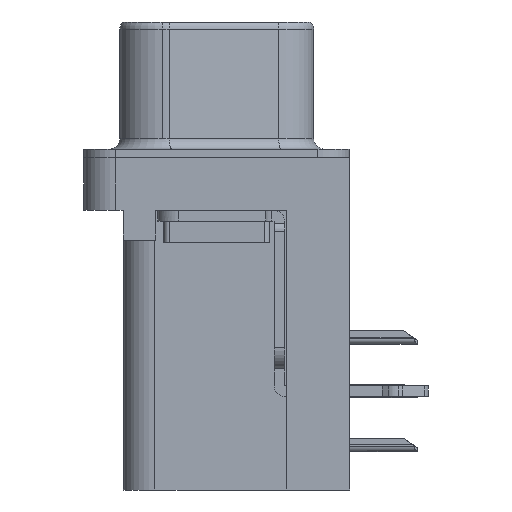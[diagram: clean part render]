
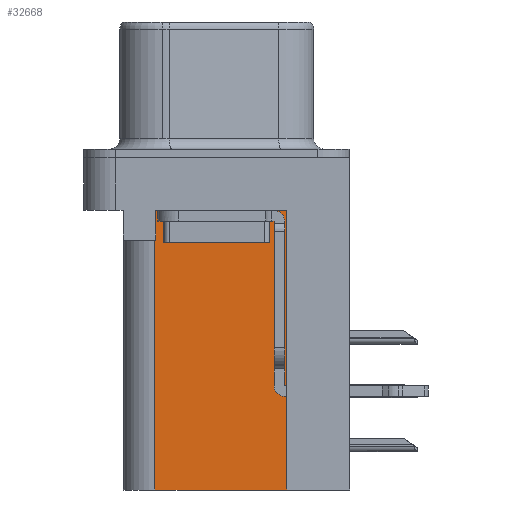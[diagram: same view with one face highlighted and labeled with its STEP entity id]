
A CAD part, left-side view. The second image highlights one B-rep face of the part: STEP entity #32668.
In plain terms, the highlighted planar face has unit normal (-1, 0, 0).
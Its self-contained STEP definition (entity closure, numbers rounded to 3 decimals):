
#428 = DIRECTION ( 'NONE',  ( 0., 1., 0. ) ) ;
#1428 = DIRECTION ( 'NONE',  ( 0., 1., 0. ) ) ;
#2313 = LINE ( 'NONE', #2747, #16010 ) ;
#2744 = CARTESIAN_POINT ( 'NONE',  ( 3.79, 2.895, -3.9 ) ) ;
#2747 = CARTESIAN_POINT ( 'NONE',  ( 3.79, 2.925, -15.7 ) ) ;
#3429 = DIRECTION ( 'NONE',  ( 0., 1., 0. ) ) ;
#3838 = VECTOR ( 'NONE', #3429, 1000. ) ;
#4020 = CARTESIAN_POINT ( 'NONE',  ( 3.79, -3.295, -15.7 ) ) ;
#4202 = EDGE_LOOP ( 'NONE', ( #34467, #12110, #12294, #6797, #34744, #28537 ) ) ;
#4486 = VERTEX_POINT ( 'NONE', #23961 ) ;
#4537 = AXIS2_PLACEMENT_3D ( 'NONE', #4020, #26140, #9547 ) ;
#5960 = VECTOR ( 'NONE', #428, 1000. ) ;
#6689 = CARTESIAN_POINT ( 'NONE',  ( 3.79, 2.895, -3.9 ) ) ;
#6797 = ORIENTED_EDGE ( 'NONE', *, *, #20792, .F. ) ;
#6993 = LINE ( 'NONE', #6689, #27405 ) ;
#8713 = VERTEX_POINT ( 'NONE', #30419 ) ;
#9253 = FACE_OUTER_BOUND ( 'NONE', #4202, .T. ) ;
#9378 = DIRECTION ( 'NONE',  ( 0., 0., -1. ) ) ;
#9547 = DIRECTION ( 'NONE',  ( 0., 0., -1. ) ) ;
#10497 = DIRECTION ( 'NONE',  ( 0., 0., 1. ) ) ;
#10613 = CARTESIAN_POINT ( 'NONE',  ( 3.79, -3.295, -15.7 ) ) ;
#11986 = LINE ( 'NONE', #17105, #3838 ) ;
#12110 = ORIENTED_EDGE ( 'NONE', *, *, #25932, .T. ) ;
#12294 = ORIENTED_EDGE ( 'NONE', *, *, #30593, .T. ) ;
#13879 = CARTESIAN_POINT ( 'NONE',  ( 3.79, 2.895, -2.5 ) ) ;
#14132 = VECTOR ( 'NONE', #1428, 1000. ) ;
#14515 = VERTEX_POINT ( 'NONE', #21530 ) ;
#15463 = LINE ( 'NONE', #10613, #22003 ) ;
#16010 = VECTOR ( 'NONE', #35980, 1000. ) ;
#16483 = CARTESIAN_POINT ( 'NONE',  ( 3.79, -3.295, -2.5 ) ) ;
#16858 = CARTESIAN_POINT ( 'NONE',  ( 3.79, -3.295, -15.7 ) ) ;
#17105 = CARTESIAN_POINT ( 'NONE',  ( 3.79, 0., -3.9 ) ) ;
#17711 = PLANE ( 'NONE',  #4537 ) ;
#17827 = CARTESIAN_POINT ( 'NONE',  ( 3.79, -3.295, -2.5 ) ) ;
#19565 = VERTEX_POINT ( 'NONE', #16483 ) ;
#20792 = EDGE_CURVE ( 'NONE', #4486, #14515, #2313, .T. ) ;
#21477 = LINE ( 'NONE', #17827, #14132 ) ;
#21530 = CARTESIAN_POINT ( 'NONE',  ( 3.79, 2.925, -3.9 ) ) ;
#22003 = VECTOR ( 'NONE', #10497, 1000. ) ;
#22671 = EDGE_CURVE ( 'NONE', #8713, #4486, #27257, .T. ) ;
#22867 = EDGE_CURVE ( 'NONE', #8713, #19565, #15463, .T. ) ;
#23961 = CARTESIAN_POINT ( 'NONE',  ( 3.79, 2.925, -15.7 ) ) ;
#25932 = EDGE_CURVE ( 'NONE', #31920, #28378, #6993, .T. ) ;
#26140 = DIRECTION ( 'NONE',  ( 1., 0., 0. ) ) ;
#27257 = LINE ( 'NONE', #16858, #5960 ) ;
#27405 = VECTOR ( 'NONE', #9378, 1000. ) ;
#28378 = VERTEX_POINT ( 'NONE', #2744 ) ;
#28537 = ORIENTED_EDGE ( 'NONE', *, *, #22867, .T. ) ;
#30419 = CARTESIAN_POINT ( 'NONE',  ( 3.79, -3.295, -15.7 ) ) ;
#30593 = EDGE_CURVE ( 'NONE', #28378, #14515, #11986, .T. ) ;
#30716 = EDGE_CURVE ( 'NONE', #19565, #31920, #21477, .T. ) ;
#31920 = VERTEX_POINT ( 'NONE', #13879 ) ;
#32668 = ADVANCED_FACE ( 'NONE', ( #9253 ), #17711, .F. ) ;
#34467 = ORIENTED_EDGE ( 'NONE', *, *, #30716, .T. ) ;
#34744 = ORIENTED_EDGE ( 'NONE', *, *, #22671, .F. ) ;
#35980 = DIRECTION ( 'NONE',  ( 0., 0., 1. ) ) ;
